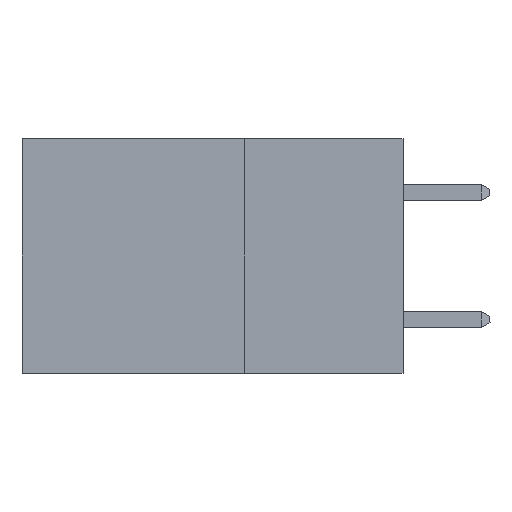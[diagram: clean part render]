
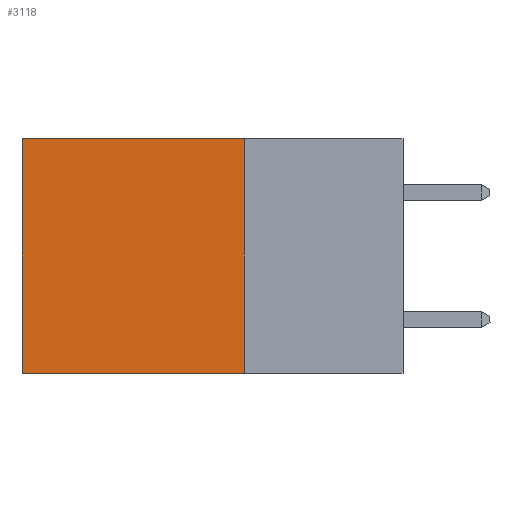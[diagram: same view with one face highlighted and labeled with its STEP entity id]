
A CAD part, left-side view. The second image highlights one B-rep face of the part: STEP entity #3118.
In plain terms, the highlighted planar face has unit normal (-1, 0, 0).
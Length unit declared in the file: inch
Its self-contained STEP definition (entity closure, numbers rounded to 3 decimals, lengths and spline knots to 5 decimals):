
#55 = DIRECTION ( 'NONE',  ( 0., 1., 0. ) ) ;
#348 = ORIENTED_EDGE ( 'NONE', *, *, #6668, .F. ) ;
#474 = EDGE_CURVE ( 'NONE', #4123, #13945, #8982, .T. ) ;
#645 = PLANE ( 'NONE',  #8232 ) ;
#3118 = ADVANCED_FACE ( 'NONE', ( #15220 ), #645, .F. ) ;
#4123 = VERTEX_POINT ( 'NONE', #7672 ) ;
#4258 = VECTOR ( 'NONE', #7478, 39.37008 ) ;
#4859 = CARTESIAN_POINT ( 'NONE',  ( 0.2875, 0.25, 0. ) ) ;
#5114 = EDGE_CURVE ( 'NONE', #17253, #13945, #5354, .T. ) ;
#5354 = LINE ( 'NONE', #5392, #13315 ) ;
#5392 = CARTESIAN_POINT ( 'NONE',  ( 0.2875, 0.25, -0.37 ) ) ;
#5422 = DIRECTION ( 'NONE',  ( 0., 1., 0. ) ) ;
#5576 = ORIENTED_EDGE ( 'NONE', *, *, #5114, .F. ) ;
#5758 = ORIENTED_EDGE ( 'NONE', *, *, #7669, .T. ) ;
#5897 = ORIENTED_EDGE ( 'NONE', *, *, #474, .T. ) ;
#5909 = VECTOR ( 'NONE', #5422, 39.37008 ) ;
#6668 = EDGE_CURVE ( 'NONE', #8941, #17253, #9431, .T. ) ;
#6963 = LINE ( 'NONE', #13448, #5909 ) ;
#7204 = DIRECTION ( 'NONE',  ( 0., 0., -1. ) ) ;
#7478 = DIRECTION ( 'NONE',  ( 0., 0., -1. ) ) ;
#7669 = EDGE_CURVE ( 'NONE', #8941, #4123, #6963, .T. ) ;
#7672 = CARTESIAN_POINT ( 'NONE',  ( 0.2875, 0.6, 0. ) ) ;
#8232 = AXIS2_PLACEMENT_3D ( 'NONE', #11388, #16702, #13978 ) ;
#8377 = CARTESIAN_POINT ( 'NONE',  ( 0.2875, 0.6, -0.37 ) ) ;
#8941 = VERTEX_POINT ( 'NONE', #4859 ) ;
#8982 = LINE ( 'NONE', #11002, #13217 ) ;
#9431 = LINE ( 'NONE', #14349, #4258 ) ;
#10566 = EDGE_LOOP ( 'NONE', ( #5897, #5576, #348, #5758 ) ) ;
#11002 = CARTESIAN_POINT ( 'NONE',  ( 0.2875, 0.6, 0. ) ) ;
#11388 = CARTESIAN_POINT ( 'NONE',  ( 0.2875, 0.25, 0. ) ) ;
#13217 = VECTOR ( 'NONE', #7204, 39.37008 ) ;
#13315 = VECTOR ( 'NONE', #55, 39.37008 ) ;
#13448 = CARTESIAN_POINT ( 'NONE',  ( 0.2875, 0.25, 0. ) ) ;
#13945 = VERTEX_POINT ( 'NONE', #8377 ) ;
#13978 = DIRECTION ( 'NONE',  ( 0., 0., -1. ) ) ;
#14349 = CARTESIAN_POINT ( 'NONE',  ( 0.2875, 0.25, 0. ) ) ;
#15220 = FACE_OUTER_BOUND ( 'NONE', #10566, .T. ) ;
#15529 = CARTESIAN_POINT ( 'NONE',  ( 0.2875, 0.25, -0.37 ) ) ;
#16702 = DIRECTION ( 'NONE',  ( 1., 0., 0. ) ) ;
#17253 = VERTEX_POINT ( 'NONE', #15529 ) ;
